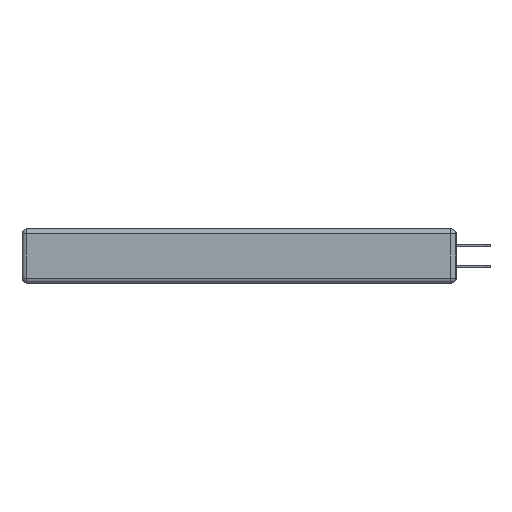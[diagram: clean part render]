
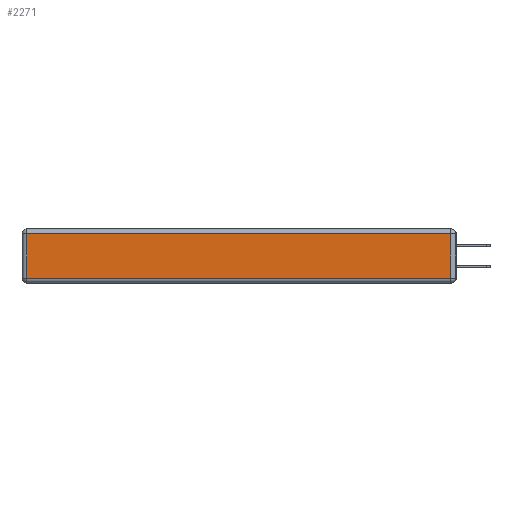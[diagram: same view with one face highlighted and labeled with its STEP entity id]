
A CAD part, left-side view. The second image highlights one B-rep face of the part: STEP entity #2271.
In plain terms, the highlighted planar face has unit normal (-1, 0, 0).
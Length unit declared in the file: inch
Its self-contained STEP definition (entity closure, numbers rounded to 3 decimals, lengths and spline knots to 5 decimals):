
#343 = ORIENTED_EDGE ( 'NONE', *, *, #5327, .T. ) ;
#519 = CARTESIAN_POINT ( 'NONE',  ( 0., 0.03, -0.313 ) ) ;
#671 = VECTOR ( 'NONE', #6696, 39.37008 ) ;
#977 = EDGE_LOOP ( 'NONE', ( #2589, #11901, #343, #11990 ) ) ;
#1608 = VECTOR ( 'NONE', #13804, 39.37008 ) ;
#2166 = VECTOR ( 'NONE', #11789, 39.37008 ) ;
#2222 = VECTOR ( 'NONE', #10951, 39.37008 ) ;
#2271 = ADVANCED_FACE ( 'NONE', ( #4883 ), #2861, .T. ) ;
#2589 = ORIENTED_EDGE ( 'NONE', *, *, #7653, .T. ) ;
#2861 = PLANE ( 'NONE',  #7290 ) ;
#3144 = CARTESIAN_POINT ( 'NONE',  ( 0., 0.03, -0.343 ) ) ;
#3343 = CARTESIAN_POINT ( 'NONE',  ( 0., 2.72, -0.343 ) ) ;
#4348 = CARTESIAN_POINT ( 'NONE',  ( 0., 0.03, -0.03 ) ) ;
#4883 = FACE_OUTER_BOUND ( 'NONE', #977, .T. ) ;
#5288 = EDGE_CURVE ( 'NONE', #11971, #8714, #12607, .T. ) ;
#5327 = EDGE_CURVE ( 'NONE', #8714, #8011, #8332, .T. ) ;
#6696 = DIRECTION ( 'NONE',  ( 0., 1., 0. ) ) ;
#7290 = AXIS2_PLACEMENT_3D ( 'NONE', #7727, #8768, #7520 ) ;
#7520 = DIRECTION ( 'NONE',  ( 0., 0., 1. ) ) ;
#7653 = EDGE_CURVE ( 'NONE', #10232, #11971, #9829, .T. ) ;
#7727 = CARTESIAN_POINT ( 'NONE',  ( 0., 0., -0.343 ) ) ;
#8011 = VERTEX_POINT ( 'NONE', #10047 ) ;
#8332 = LINE ( 'NONE', #14934, #671 ) ;
#8714 = VERTEX_POINT ( 'NONE', #4348 ) ;
#8768 = DIRECTION ( 'NONE',  ( -1., 0., 0. ) ) ;
#9350 = CARTESIAN_POINT ( 'NONE',  ( 0., 0., -0.313 ) ) ;
#9829 = LINE ( 'NONE', #9350, #2166 ) ;
#10047 = CARTESIAN_POINT ( 'NONE',  ( 0., 2.72, -0.03 ) ) ;
#10155 = CARTESIAN_POINT ( 'NONE',  ( 0., 2.72, -0.313 ) ) ;
#10232 = VERTEX_POINT ( 'NONE', #10155 ) ;
#10951 = DIRECTION ( 'NONE',  ( 0., 0., -1. ) ) ;
#11789 = DIRECTION ( 'NONE',  ( 0., -1., 0. ) ) ;
#11901 = ORIENTED_EDGE ( 'NONE', *, *, #5288, .T. ) ;
#11971 = VERTEX_POINT ( 'NONE', #519 ) ;
#11990 = ORIENTED_EDGE ( 'NONE', *, *, #15283, .T. ) ;
#12123 = LINE ( 'NONE', #3343, #2222 ) ;
#12607 = LINE ( 'NONE', #3144, #1608 ) ;
#13804 = DIRECTION ( 'NONE',  ( 0., 0., 1. ) ) ;
#14934 = CARTESIAN_POINT ( 'NONE',  ( 0., 2.75, -0.03 ) ) ;
#15283 = EDGE_CURVE ( 'NONE', #8011, #10232, #12123, .T. ) ;
